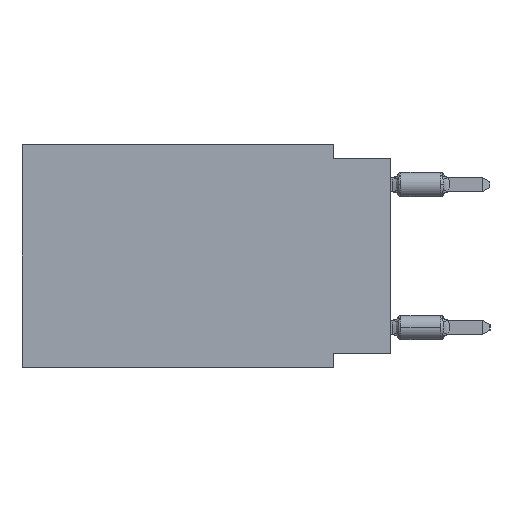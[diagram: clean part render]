
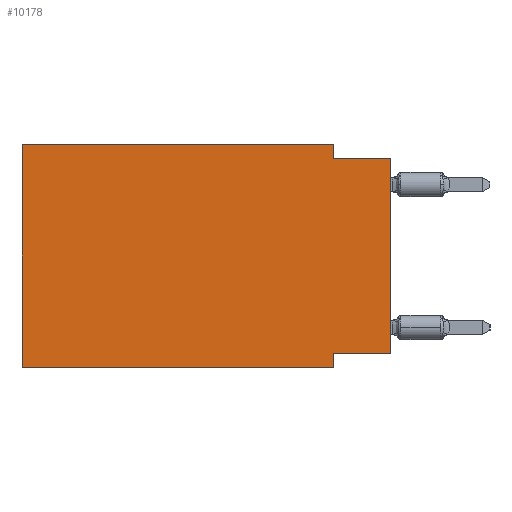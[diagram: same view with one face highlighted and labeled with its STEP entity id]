
A CAD part, left-side view. The second image highlights one B-rep face of the part: STEP entity #10178.
In plain terms, the highlighted planar face has unit normal (-1, 0, 0).
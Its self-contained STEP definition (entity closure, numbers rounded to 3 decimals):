
#213 = EDGE_LOOP ( 'NONE', ( #43080, #13888, #26870, #24653, #34602, #15841, #18020, #17278 ) ) ;
#948 = DIRECTION ( 'NONE',  ( 0., -1., 0. ) ) ;
#1898 = VERTEX_POINT ( 'NONE', #27617 ) ;
#2193 = CARTESIAN_POINT ( 'NONE',  ( 0., 2.54, 0. ) ) ;
#2377 = CARTESIAN_POINT ( 'NONE',  ( 0., 0., -0.635 ) ) ;
#6280 = FACE_OUTER_BOUND ( 'NONE', #213, .T. ) ;
#7436 = DIRECTION ( 'NONE',  ( 0., 0., -1. ) ) ;
#7937 = VERTEX_POINT ( 'NONE', #35231 ) ;
#8166 = DIRECTION ( 'NONE',  ( 0., -1., 0. ) ) ;
#8390 = LINE ( 'NONE', #2193, #31428 ) ;
#9415 = VERTEX_POINT ( 'NONE', #33867 ) ;
#9474 = DIRECTION ( 'NONE',  ( 1., 0., 0. ) ) ;
#10178 = ADVANCED_FACE ( 'NONE', ( #6280 ), #16777, .F. ) ;
#10623 = LINE ( 'NONE', #14489, #15303 ) ;
#11826 = LINE ( 'NONE', #2377, #22895 ) ;
#13537 = CARTESIAN_POINT ( 'NONE',  ( 0., 2.54, 0. ) ) ;
#13888 = ORIENTED_EDGE ( 'NONE', *, *, #42941, .F. ) ;
#14225 = VERTEX_POINT ( 'NONE', #42902 ) ;
#14489 = CARTESIAN_POINT ( 'NONE',  ( 0., 2.54, -9.906 ) ) ;
#14556 = DIRECTION ( 'NONE',  ( 0., 1., 0. ) ) ;
#15303 = VECTOR ( 'NONE', #7436, 1000. ) ;
#15513 = EDGE_CURVE ( 'NONE', #44434, #7937, #42909, .T. ) ;
#15705 = VECTOR ( 'NONE', #39493, 1000. ) ;
#15841 = ORIENTED_EDGE ( 'NONE', *, *, #32673, .T. ) ;
#16133 = LINE ( 'NONE', #30087, #40020 ) ;
#16777 = PLANE ( 'NONE',  #34470 ) ;
#17278 = ORIENTED_EDGE ( 'NONE', *, *, #28198, .F. ) ;
#17795 = EDGE_CURVE ( 'NONE', #30090, #14225, #16133, .T. ) ;
#18020 = ORIENTED_EDGE ( 'NONE', *, *, #27342, .F. ) ;
#18543 = CARTESIAN_POINT ( 'NONE',  ( 0., 16.383, -9.906 ) ) ;
#19919 = VERTEX_POINT ( 'NONE', #20727 ) ;
#20727 = CARTESIAN_POINT ( 'NONE',  ( 0., 2.54, -0.635 ) ) ;
#20732 = VERTEX_POINT ( 'NONE', #13537 ) ;
#20924 = DIRECTION ( 'NONE',  ( 0., -1., 0. ) ) ;
#21086 = VECTOR ( 'NONE', #948, 1000. ) ;
#22895 = VECTOR ( 'NONE', #8166, 1000. ) ;
#23441 = DIRECTION ( 'NONE',  ( 0., 0., -1. ) ) ;
#24653 = ORIENTED_EDGE ( 'NONE', *, *, #44464, .F. ) ;
#24822 = LINE ( 'NONE', #30987, #30279 ) ;
#25190 = LINE ( 'NONE', #18543, #21086 ) ;
#25306 = CARTESIAN_POINT ( 'NONE',  ( 0., 0., -9.271 ) ) ;
#25549 = CARTESIAN_POINT ( 'NONE',  ( 0., 16.383, 0. ) ) ;
#25632 = CARTESIAN_POINT ( 'NONE',  ( 0., 0., -9.271 ) ) ;
#26870 = ORIENTED_EDGE ( 'NONE', *, *, #28288, .F. ) ;
#27342 = EDGE_CURVE ( 'NONE', #1898, #9415, #10623, .T. ) ;
#27617 = CARTESIAN_POINT ( 'NONE',  ( 0., 2.54, -9.271 ) ) ;
#28198 = EDGE_CURVE ( 'NONE', #30090, #1898, #28945, .T. ) ;
#28288 = EDGE_CURVE ( 'NONE', #20732, #19919, #8390, .T. ) ;
#28945 = LINE ( 'NONE', #25306, #42402 ) ;
#30087 = CARTESIAN_POINT ( 'NONE',  ( 0., 0., 0. ) ) ;
#30090 = VERTEX_POINT ( 'NONE', #25632 ) ;
#30279 = VECTOR ( 'NONE', #20924, 1000. ) ;
#30987 = CARTESIAN_POINT ( 'NONE',  ( 0., 16.383, 0. ) ) ;
#31428 = VECTOR ( 'NONE', #36485, 1000. ) ;
#32673 = EDGE_CURVE ( 'NONE', #44434, #9415, #25190, .T. ) ;
#33867 = CARTESIAN_POINT ( 'NONE',  ( 0., 2.54, -9.906 ) ) ;
#34470 = AXIS2_PLACEMENT_3D ( 'NONE', #41241, #9474, #23441 ) ;
#34602 = ORIENTED_EDGE ( 'NONE', *, *, #15513, .F. ) ;
#35231 = CARTESIAN_POINT ( 'NONE',  ( 0., 16.383, 0. ) ) ;
#36485 = DIRECTION ( 'NONE',  ( 0., 0., -1. ) ) ;
#38303 = CARTESIAN_POINT ( 'NONE',  ( 0., 16.383, -9.906 ) ) ;
#39493 = DIRECTION ( 'NONE',  ( 0., 0., 1. ) ) ;
#40020 = VECTOR ( 'NONE', #44040, 1000. ) ;
#41241 = CARTESIAN_POINT ( 'NONE',  ( 0., 16.383, 0. ) ) ;
#42402 = VECTOR ( 'NONE', #14556, 1000. ) ;
#42902 = CARTESIAN_POINT ( 'NONE',  ( 0., 0., -0.635 ) ) ;
#42909 = LINE ( 'NONE', #25549, #15705 ) ;
#42941 = EDGE_CURVE ( 'NONE', #19919, #14225, #11826, .T. ) ;
#43080 = ORIENTED_EDGE ( 'NONE', *, *, #17795, .T. ) ;
#44040 = DIRECTION ( 'NONE',  ( 0., 0., 1. ) ) ;
#44434 = VERTEX_POINT ( 'NONE', #38303 ) ;
#44464 = EDGE_CURVE ( 'NONE', #7937, #20732, #24822, .T. ) ;
